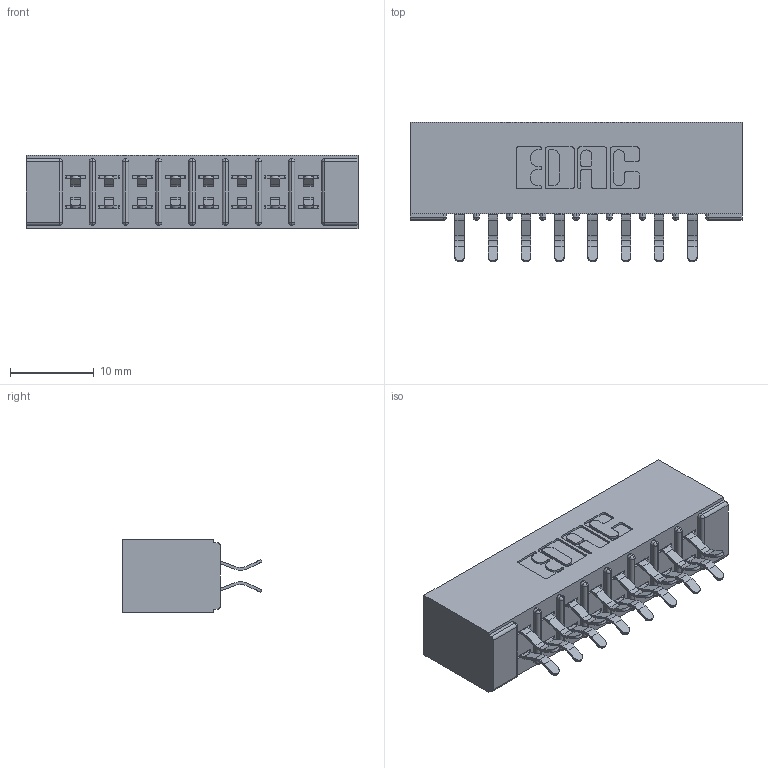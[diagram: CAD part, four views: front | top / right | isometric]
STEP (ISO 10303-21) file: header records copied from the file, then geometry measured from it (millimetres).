
FILE_DESCRIPTION (( 'STEP AP203' ), '1' );
FILE_NAME ('305-016-556-501.STEP', '2019-09-09T12:26:38', ( '' ), ( '' ), 'SwSTEP 2.0', 'SolidWorks 2016', '' );
FILE_SCHEMA (( 'CONFIG_CONTROL_DESIGN' ));
Length unit declared in the file: inch
Products named in the file (3): 305 Part_No Mounting; 305-016-556-501; 305-290-001_556
Assembly tree (17 placements, depth 2):
  305-016-556-501
    305 Part_No Mounting
    305-290-001_556  x16
Bounding box: 39.57 x 16.64 x 8.71 mm (x, y, z)
Volume: 2572.7 mm3; surface area: 4877.4 mm2
Topology: 17 solids, 17 shells, 1004 faces, 2876 edges, 1872 vertices
Faces by surface type: plane 560, cylinder 412, sphere 32
Entity records: 12745 total; most frequent: CARTESIAN_POINT 2110, ORIENTED_EDGE 2088, DIRECTION 2070, EDGE_CURVE 1044, VECTOR 806, LINE 806, VERTEX_POINT 672, AXIS2_PLACEMENT_3D 632
